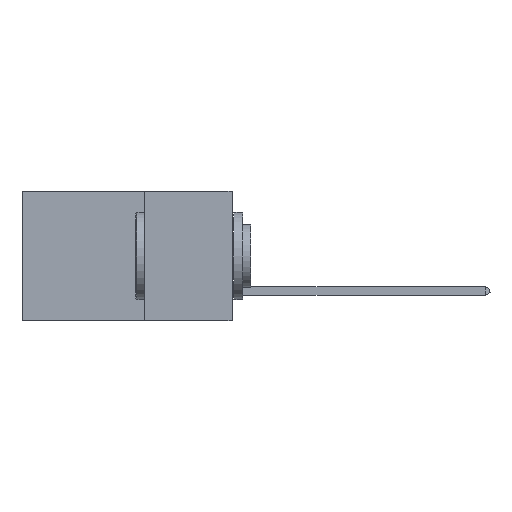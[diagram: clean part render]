
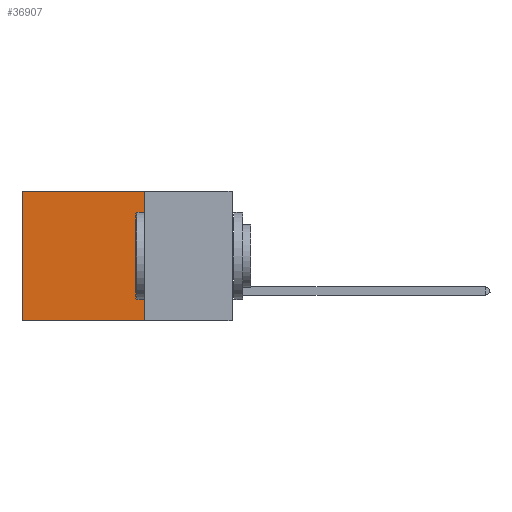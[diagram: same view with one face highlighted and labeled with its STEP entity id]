
A CAD part, left-side view. The second image highlights one B-rep face of the part: STEP entity #36907.
In plain terms, the highlighted planar face has unit normal (-1, 0, 0).
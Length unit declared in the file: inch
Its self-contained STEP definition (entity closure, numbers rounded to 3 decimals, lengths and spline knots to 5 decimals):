
#122 = EDGE_CURVE ( 'NONE', #22196, #15886, #4371, .T. ) ;
#1007 = VERTEX_POINT ( 'NONE', #14347 ) ;
#3065 = ORIENTED_EDGE ( 'NONE', *, *, #30100, .F. ) ;
#3546 = ORIENTED_EDGE ( 'NONE', *, *, #13966, .T. ) ;
#4371 = LINE ( 'NONE', #25953, #24032 ) ;
#4773 = CARTESIAN_POINT ( 'NONE',  ( 0.2875, 0.25, 0. ) ) ;
#7384 = CARTESIAN_POINT ( 'NONE',  ( 0.2875, 0.25, -0.37 ) ) ;
#7542 = LINE ( 'NONE', #11729, #43802 ) ;
#7831 = CARTESIAN_POINT ( 'NONE',  ( 0.2875, 0.25, 0. ) ) ;
#9814 = ORIENTED_EDGE ( 'NONE', *, *, #25233, .T. ) ;
#10561 = AXIS2_PLACEMENT_3D ( 'NONE', #4773, #21380, #18140 ) ;
#11729 = CARTESIAN_POINT ( 'NONE',  ( 0.2875, 0.25, 0. ) ) ;
#13469 = VERTEX_POINT ( 'NONE', #25507 ) ;
#13623 = ORIENTED_EDGE ( 'NONE', *, *, #122, .F. ) ;
#13966 = EDGE_CURVE ( 'NONE', #22196, #13469, #7542, .T. ) ;
#14303 = FACE_OUTER_BOUND ( 'NONE', #32164, .T. ) ;
#14347 = CARTESIAN_POINT ( 'NONE',  ( 0.2875, 0.6, -0.37 ) ) ;
#15371 = VECTOR ( 'NONE', #39857, 39.37008 ) ;
#15886 = VERTEX_POINT ( 'NONE', #7384 ) ;
#17570 = VECTOR ( 'NONE', #33250, 39.37008 ) ;
#17985 = PLANE ( 'NONE',  #10561 ) ;
#18140 = DIRECTION ( 'NONE',  ( 0., 0., -1. ) ) ;
#18669 = LINE ( 'NONE', #43695, #17570 ) ;
#21380 = DIRECTION ( 'NONE',  ( 1., 0., 0. ) ) ;
#22196 = VERTEX_POINT ( 'NONE', #7831 ) ;
#24032 = VECTOR ( 'NONE', #35638, 39.37008 ) ;
#25233 = EDGE_CURVE ( 'NONE', #13469, #1007, #39368, .T. ) ;
#25507 = CARTESIAN_POINT ( 'NONE',  ( 0.2875, 0.6, 0. ) ) ;
#25953 = CARTESIAN_POINT ( 'NONE',  ( 0.2875, 0.25, 0. ) ) ;
#26606 = CARTESIAN_POINT ( 'NONE',  ( 0.2875, 0.6, 0. ) ) ;
#28081 = DIRECTION ( 'NONE',  ( 0., 1., 0. ) ) ;
#30100 = EDGE_CURVE ( 'NONE', #15886, #1007, #18669, .T. ) ;
#32164 = EDGE_LOOP ( 'NONE', ( #9814, #3065, #13623, #3546 ) ) ;
#33250 = DIRECTION ( 'NONE',  ( 0., 1., 0. ) ) ;
#35638 = DIRECTION ( 'NONE',  ( 0., 0., -1. ) ) ;
#36907 = ADVANCED_FACE ( 'NONE', ( #14303 ), #17985, .F. ) ;
#39368 = LINE ( 'NONE', #26606, #15371 ) ;
#39857 = DIRECTION ( 'NONE',  ( 0., 0., -1. ) ) ;
#43695 = CARTESIAN_POINT ( 'NONE',  ( 0.2875, 0.25, -0.37 ) ) ;
#43802 = VECTOR ( 'NONE', #28081, 39.37008 ) ;
